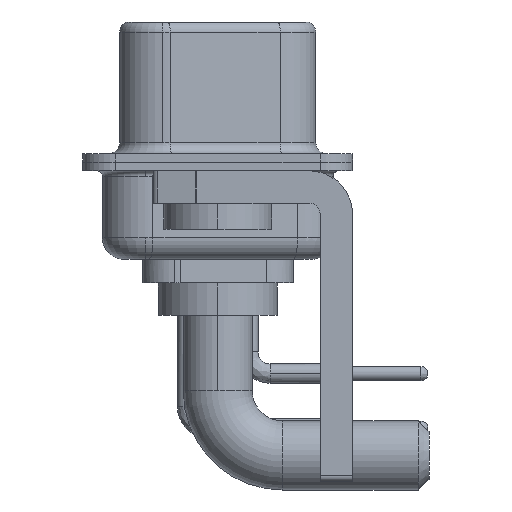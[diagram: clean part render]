
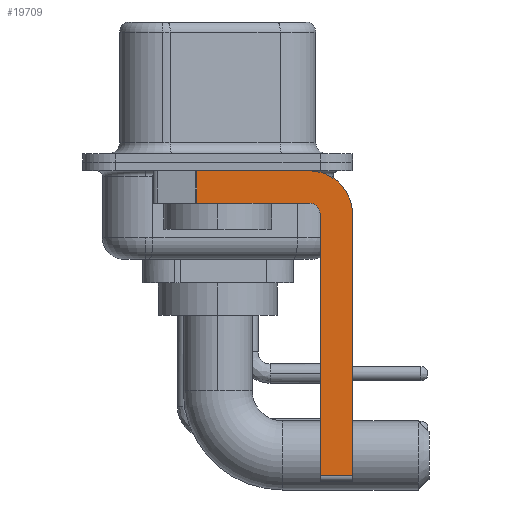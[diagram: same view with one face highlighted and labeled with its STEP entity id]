
A CAD part, left-side view. The second image highlights one B-rep face of the part: STEP entity #19709.
In plain terms, the highlighted planar face has unit normal (-1, 0, 0).
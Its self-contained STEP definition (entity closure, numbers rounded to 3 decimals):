
#255 = VECTOR ( 'NONE', #17451, 1000. ) ;
#943 = VECTOR ( 'NONE', #24797, 1000. ) ;
#996 = ORIENTED_EDGE ( 'NONE', *, *, #6463, .F. ) ;
#1146 = DIRECTION ( 'NONE',  ( -1., 0., 0. ) ) ;
#3007 = DIRECTION ( 'NONE',  ( 0., 0., -1. ) ) ;
#3153 = DIRECTION ( 'NONE',  ( 0., 0., -1. ) ) ;
#3327 = ORIENTED_EDGE ( 'NONE', *, *, #4938, .F. ) ;
#3466 = VERTEX_POINT ( 'NONE', #11074 ) ;
#3541 = LINE ( 'NONE', #11481, #255 ) ;
#3618 = CARTESIAN_POINT ( 'NONE',  ( -2.9, -4.25, -2.4 ) ) ;
#3749 = VERTEX_POINT ( 'NONE', #24711 ) ;
#3773 = DIRECTION ( 'NONE',  ( 0., -1., 0. ) ) ;
#4039 = CARTESIAN_POINT ( 'NONE',  ( -2.9, -6.25, -2.4 ) ) ;
#4069 = DIRECTION ( 'NONE',  ( 1., 0., 0. ) ) ;
#4121 = EDGE_CURVE ( 'NONE', #25564, #20568, #12632, .T. ) ;
#4938 = EDGE_CURVE ( 'NONE', #18011, #14459, #23528, .T. ) ;
#5200 = CARTESIAN_POINT ( 'NONE',  ( -2.9, -4.75, -14.8 ) ) ;
#5733 = CARTESIAN_POINT ( 'NONE',  ( -2.9, 3., -0.4 ) ) ;
#6463 = EDGE_CURVE ( 'NONE', #19187, #3466, #23911, .T. ) ;
#7073 = VECTOR ( 'NONE', #3153, 1000. ) ;
#7107 = DIRECTION ( 'NONE',  ( 0., 0., 1. ) ) ;
#7236 = EDGE_CURVE ( 'NONE', #3749, #7786, #17097, .T. ) ;
#7786 = VERTEX_POINT ( 'NONE', #9684 ) ;
#8204 = EDGE_CURVE ( 'NONE', #3466, #18011, #10692, .T. ) ;
#9052 = CARTESIAN_POINT ( 'NONE',  ( -2.9, -4.25, -1.9 ) ) ;
#9684 = CARTESIAN_POINT ( 'NONE',  ( -2.9, 0.978, -1.9 ) ) ;
#9730 = VECTOR ( 'NONE', #19643, 1000. ) ;
#10058 = PLANE ( 'NONE',  #18970 ) ;
#10187 = CARTESIAN_POINT ( 'NONE',  ( -2.9, -4.25, -2.4 ) ) ;
#10692 = CIRCLE ( 'NONE', #13983, 2. ) ;
#11074 = CARTESIAN_POINT ( 'NONE',  ( -2.9, -4.25, -0.4 ) ) ;
#11481 = CARTESIAN_POINT ( 'NONE',  ( -2.9, -4.25, -14.55 ) ) ;
#11557 = DIRECTION ( 'NONE',  ( 1., 0., 0. ) ) ;
#12015 = EDGE_CURVE ( 'NONE', #19187, #7786, #25095, .T. ) ;
#12632 = LINE ( 'NONE', #5200, #943 ) ;
#12969 = CARTESIAN_POINT ( 'NONE',  ( -2.9, -4.25, -2.4 ) ) ;
#13123 = ORIENTED_EDGE ( 'NONE', *, *, #8204, .F. ) ;
#13983 = AXIS2_PLACEMENT_3D ( 'NONE', #3618, #11557, #3007 ) ;
#14310 = EDGE_LOOP ( 'NONE', ( #996, #18705, #19519, #16294, #21720, #18266, #3327, #13123 ) ) ;
#14459 = VERTEX_POINT ( 'NONE', #21755 ) ;
#14788 = VECTOR ( 'NONE', #16964, 1000. ) ;
#15114 = CARTESIAN_POINT ( 'NONE',  ( -2.9, -4.75, -14.55 ) ) ;
#16294 = ORIENTED_EDGE ( 'NONE', *, *, #21896, .F. ) ;
#16964 = DIRECTION ( 'NONE',  ( 0., 1., 0. ) ) ;
#17097 = LINE ( 'NONE', #9052, #14788 ) ;
#17451 = DIRECTION ( 'NONE',  ( 0., -1., 0. ) ) ;
#18011 = VERTEX_POINT ( 'NONE', #22596 ) ;
#18012 = CARTESIAN_POINT ( 'NONE',  ( -2.9, 0.978, -0.4 ) ) ;
#18204 = EDGE_CURVE ( 'NONE', #25564, #14459, #3541, .T. ) ;
#18266 = ORIENTED_EDGE ( 'NONE', *, *, #18204, .T. ) ;
#18705 = ORIENTED_EDGE ( 'NONE', *, *, #12015, .T. ) ;
#18929 = VECTOR ( 'NONE', #3773, 1000. ) ;
#18970 = AXIS2_PLACEMENT_3D ( 'NONE', #10187, #4069, #19802 ) ;
#19125 = CARTESIAN_POINT ( 'NONE',  ( -2.9, 0.978, -1.9 ) ) ;
#19187 = VERTEX_POINT ( 'NONE', #18012 ) ;
#19519 = ORIENTED_EDGE ( 'NONE', *, *, #7236, .F. ) ;
#19643 = DIRECTION ( 'NONE',  ( 0., 0., -1. ) ) ;
#19709 = ADVANCED_FACE ( 'NONE', ( #21873 ), #10058, .F. ) ;
#19802 = DIRECTION ( 'NONE',  ( 0., 0., -1. ) ) ;
#19931 = CIRCLE ( 'NONE', #23670, 0.5 ) ;
#20568 = VERTEX_POINT ( 'NONE', #22718 ) ;
#21720 = ORIENTED_EDGE ( 'NONE', *, *, #4121, .F. ) ;
#21755 = CARTESIAN_POINT ( 'NONE',  ( -2.9, -6.25, -14.55 ) ) ;
#21873 = FACE_OUTER_BOUND ( 'NONE', #14310, .T. ) ;
#21896 = EDGE_CURVE ( 'NONE', #20568, #3749, #19931, .T. ) ;
#22596 = CARTESIAN_POINT ( 'NONE',  ( -2.9, -6.25, -2.4 ) ) ;
#22718 = CARTESIAN_POINT ( 'NONE',  ( -2.9, -4.75, -2.4 ) ) ;
#23528 = LINE ( 'NONE', #4039, #9730 ) ;
#23670 = AXIS2_PLACEMENT_3D ( 'NONE', #12969, #1146, #7107 ) ;
#23911 = LINE ( 'NONE', #5733, #18929 ) ;
#24711 = CARTESIAN_POINT ( 'NONE',  ( -2.9, -4.25, -1.9 ) ) ;
#24797 = DIRECTION ( 'NONE',  ( 0., 0., 1. ) ) ;
#25095 = LINE ( 'NONE', #19125, #7073 ) ;
#25564 = VERTEX_POINT ( 'NONE', #15114 ) ;
